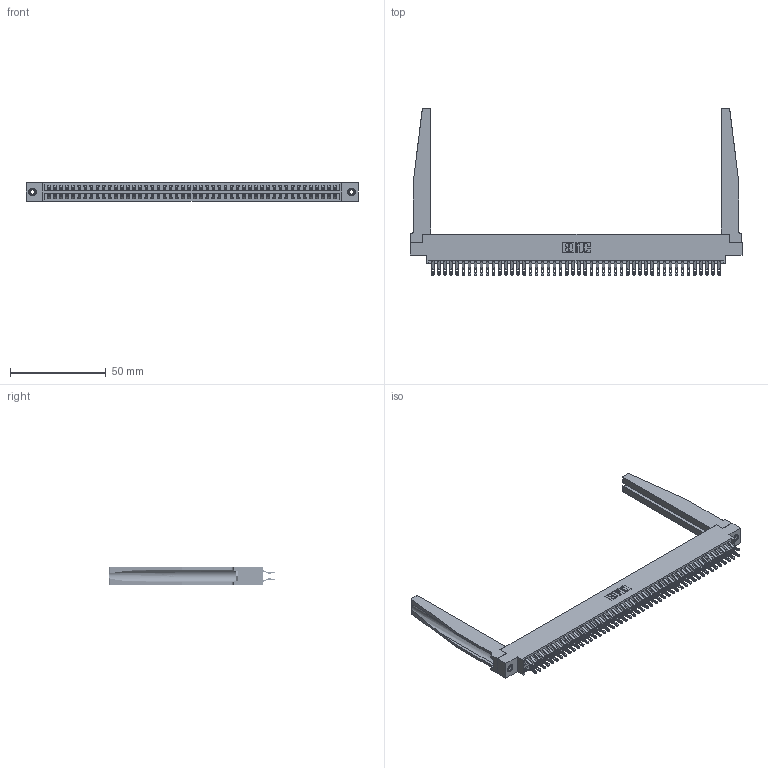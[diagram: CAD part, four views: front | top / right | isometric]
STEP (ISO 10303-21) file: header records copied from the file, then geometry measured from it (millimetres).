
FILE_DESCRIPTION (( 'STEP AP203' ), '1' );
FILE_NAME ('346-096-555-878.STEP', '2022-05-26T16:48:31', ( '' ), ( '' ), 'SwSTEP 2.0', 'SolidWorks 2020', '' );
FILE_SCHEMA (( 'CONFIG_CONTROL_DESIGN' ));
Length unit declared in the file: inch
Products named in the file (5): 346 Part_0.170 Offset - 0.156 Dia-TH; 346-096-555-878; 346-220-078_345-220-078; 345-292-001_555 Tail; 345-250-001_345-250-001-102
Assembly tree (101 placements, depth 2):
  346-096-555-878
    346 Part_0.170 Offset - 0.156 Dia-TH
    345-292-001_555 Tail  x96
    346-220-078_345-220-078  x2
    345-250-001_345-250-001-102  x2
Bounding box: 172.97 x 86.74 x 9.4 mm (x, y, z)
Volume: 23928.3 mm3; surface area: 31233 mm2
Topology: 101 solids, 101 shells, 5942 faces, 18553 edges, 12358 vertices
Faces by surface type: plane 3404, cylinder 2486, bspline 36, cone 12, torus 4
Entity records: 36140 total; most frequent: CARTESIAN_POINT 6927, ORIENTED_EDGE 5718, DIRECTION 5109, EDGE_CURVE 2859, VECTOR 2421, LINE 2421, VERTEX_POINT 1900, AXIS2_PLACEMENT_3D 1344
